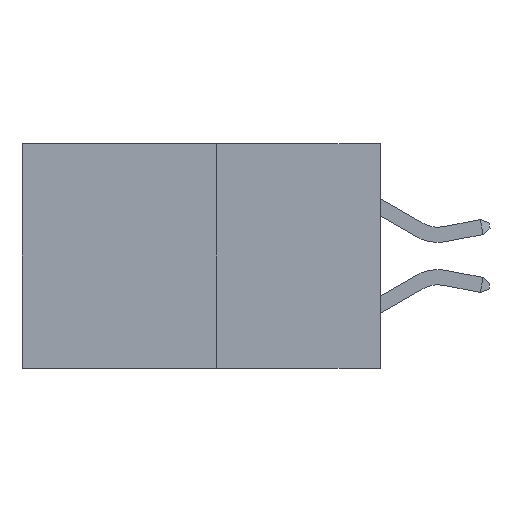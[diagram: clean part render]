
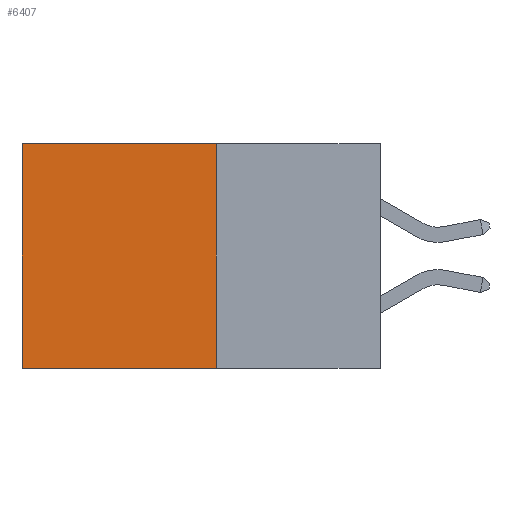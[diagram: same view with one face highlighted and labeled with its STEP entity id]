
A CAD part, left-side view. The second image highlights one B-rep face of the part: STEP entity #6407.
In plain terms, the highlighted planar face has unit normal (-1, 0, 0).
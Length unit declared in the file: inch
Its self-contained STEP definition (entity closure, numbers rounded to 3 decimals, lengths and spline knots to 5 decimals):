
#19 = LINE ( 'NONE', #14479, #5954 ) ;
#434 = CARTESIAN_POINT ( 'NONE',  ( 0.277, 0.59, 0. ) ) ;
#1295 = EDGE_CURVE ( 'NONE', #14151, #14110, #4586, .T. ) ;
#2759 = CARTESIAN_POINT ( 'NONE',  ( 0.277, 0.59, -0.37 ) ) ;
#2812 = CARTESIAN_POINT ( 'NONE',  ( 0.277, 0.27, 0. ) ) ;
#3323 = CARTESIAN_POINT ( 'NONE',  ( 0.277, 0.59, -0.37 ) ) ;
#4238 = LINE ( 'NONE', #2759, #13234 ) ;
#4366 = ORIENTED_EDGE ( 'NONE', *, *, #9396, .F. ) ;
#4586 = LINE ( 'NONE', #4656, #7079 ) ;
#4656 = CARTESIAN_POINT ( 'NONE',  ( 0.277, 0.27, 0. ) ) ;
#5278 = DIRECTION ( 'NONE',  ( 0., 1., 0. ) ) ;
#5458 = FACE_OUTER_BOUND ( 'NONE', #13922, .T. ) ;
#5954 = VECTOR ( 'NONE', #5278, 39.37008 ) ;
#6307 = CARTESIAN_POINT ( 'NONE',  ( 0.277, 0.27, -0.37 ) ) ;
#6407 = ADVANCED_FACE ( 'NONE', ( #5458 ), #11502, .F. ) ;
#6937 = ORIENTED_EDGE ( 'NONE', *, *, #1295, .T. ) ;
#6949 = ORIENTED_EDGE ( 'NONE', *, *, #11477, .F. ) ;
#7079 = VECTOR ( 'NONE', #11357, 39.37008 ) ;
#7790 = CARTESIAN_POINT ( 'NONE',  ( 0.277, 0.27, -0.37 ) ) ;
#9004 = DIRECTION ( 'NONE',  ( 0., 0., -1. ) ) ;
#9030 = LINE ( 'NONE', #7790, #13924 ) ;
#9253 = VERTEX_POINT ( 'NONE', #6307 ) ;
#9316 = EDGE_CURVE ( 'NONE', #14110, #14707, #4238, .T. ) ;
#9396 = EDGE_CURVE ( 'NONE', #9253, #14707, #19, .T. ) ;
#9963 = DIRECTION ( 'NONE',  ( 0., 0., -1. ) ) ;
#11357 = DIRECTION ( 'NONE',  ( 0., 1., 0. ) ) ;
#11442 = DIRECTION ( 'NONE',  ( 0., 0., -1. ) ) ;
#11469 = DIRECTION ( 'NONE',  ( 1., 0., 0. ) ) ;
#11477 = EDGE_CURVE ( 'NONE', #14151, #9253, #9030, .T. ) ;
#11502 = PLANE ( 'NONE',  #14184 ) ;
#11602 = CARTESIAN_POINT ( 'NONE',  ( 0.277, 0.27, -0.37 ) ) ;
#13234 = VECTOR ( 'NONE', #9963, 39.37008 ) ;
#13922 = EDGE_LOOP ( 'NONE', ( #14885, #4366, #6949, #6937 ) ) ;
#13924 = VECTOR ( 'NONE', #9004, 39.37008 ) ;
#14110 = VERTEX_POINT ( 'NONE', #434 ) ;
#14151 = VERTEX_POINT ( 'NONE', #2812 ) ;
#14184 = AXIS2_PLACEMENT_3D ( 'NONE', #11602, #11469, #11442 ) ;
#14479 = CARTESIAN_POINT ( 'NONE',  ( 0.277, 0.27, -0.37 ) ) ;
#14707 = VERTEX_POINT ( 'NONE', #3323 ) ;
#14885 = ORIENTED_EDGE ( 'NONE', *, *, #9316, .T. ) ;
